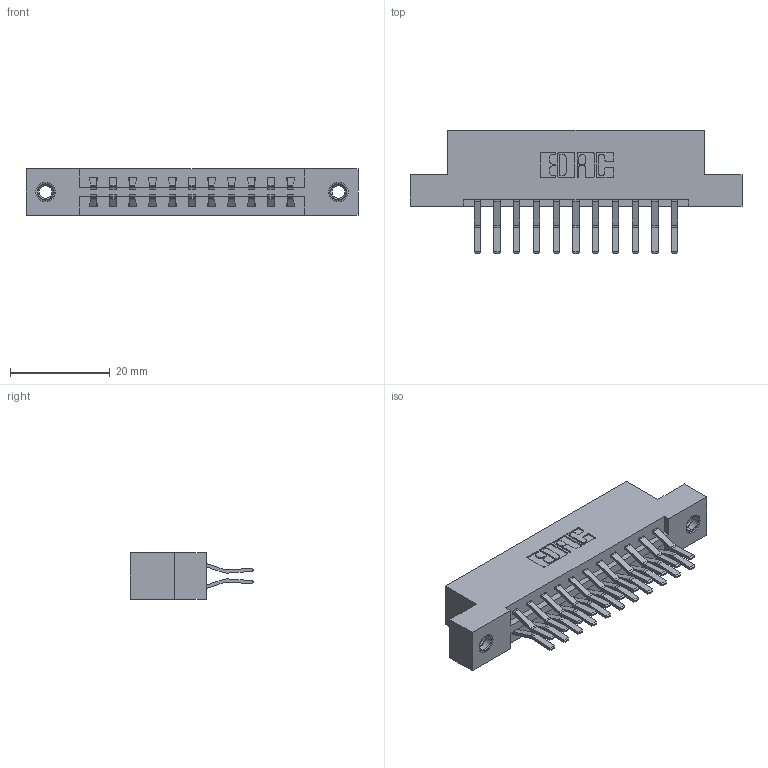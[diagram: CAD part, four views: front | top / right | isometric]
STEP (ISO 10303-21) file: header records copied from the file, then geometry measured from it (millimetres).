
FILE_DESCRIPTION (( 'STEP AP203' ), '1' );
FILE_NAME ('387-022-560-207.STEP', '2019-10-16T17:34:31', ( '' ), ( '' ), 'SwSTEP 2.0', 'SolidWorks 2016', '' );
FILE_SCHEMA (( 'CONFIG_CONTROL_DESIGN' ));
Length unit declared in the file: inch
Products named in the file (4): 387-022-560-207; 337 Part_Flush Mounting Lugs - 0.156 Dia-TI; 345-250-001_345-250-005-103; 345-292-001_560 Tail
Assembly tree (25 placements, depth 2):
  387-022-560-207
    337 Part_Flush Mounting Lugs - 0.156 Dia-TI
    345-292-001_560 Tail  x22
    345-250-001_345-250-005-103  x2
Bounding box: 66.6 x 24.78 x 9.4 mm (x, y, z)
Volume: 6736.8 mm3; surface area: 7768.1 mm2
Topology: 25 solids, 25 shells, 1406 faces, 4121 edges, 2710 vertices
Faces by surface type: plane 938, cylinder 452, cone 12, torus 4
Entity records: 13812 total; most frequent: CARTESIAN_POINT 2333, ORIENTED_EDGE 2262, DIRECTION 2077, EDGE_CURVE 1131, LINE 979, VECTOR 979, VERTEX_POINT 748, AXIS2_PLACEMENT_3D 549
